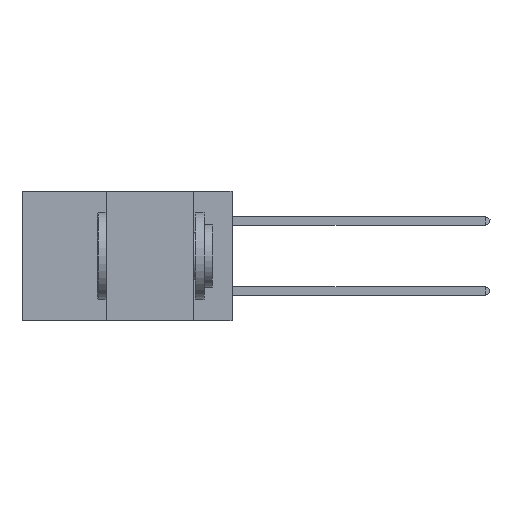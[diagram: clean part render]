
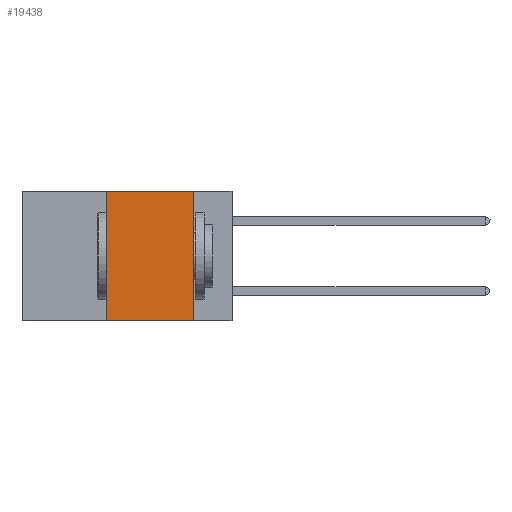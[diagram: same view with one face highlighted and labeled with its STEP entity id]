
A CAD part, left-side view. The second image highlights one B-rep face of the part: STEP entity #19438.
In plain terms, the highlighted planar face has unit normal (-1, 0, 0).
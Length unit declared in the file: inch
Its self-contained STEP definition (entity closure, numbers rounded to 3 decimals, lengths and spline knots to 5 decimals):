
#552 = CARTESIAN_POINT ( 'NONE',  ( 0., 0.11, 0. ) ) ;
#2005 = VERTEX_POINT ( 'NONE', #35096 ) ;
#2149 = VECTOR ( 'NONE', #7782, 39.37008 ) ;
#2191 = EDGE_CURVE ( 'NONE', #21267, #2005, #26869, .T. ) ;
#2265 = DIRECTION ( 'NONE',  ( 0., -1., 0. ) ) ;
#4194 = VECTOR ( 'NONE', #19752, 39.37008 ) ;
#6400 = LINE ( 'NONE', #44155, #4194 ) ;
#6740 = ORIENTED_EDGE ( 'NONE', *, *, #28919, .F. ) ;
#7676 = ORIENTED_EDGE ( 'NONE', *, *, #35363, .F. ) ;
#7782 = DIRECTION ( 'NONE',  ( 0., 0., -1. ) ) ;
#9623 = VECTOR ( 'NONE', #2265, 39.37008 ) ;
#10686 = LINE ( 'NONE', #26790, #9623 ) ;
#11464 = LINE ( 'NONE', #552, #2149 ) ;
#15037 = CARTESIAN_POINT ( 'NONE',  ( 0., 0.36, 0. ) ) ;
#16605 = AXIS2_PLACEMENT_3D ( 'NONE', #36214, #18784, #43182 ) ;
#17268 = VERTEX_POINT ( 'NONE', #19667 ) ;
#18784 = DIRECTION ( 'NONE',  ( 1., 0., 0. ) ) ;
#18826 = CARTESIAN_POINT ( 'NONE',  ( 0., 0.36, -0.37 ) ) ;
#19438 = ADVANCED_FACE ( 'NONE', ( #27217 ), #29230, .F. ) ;
#19667 = CARTESIAN_POINT ( 'NONE',  ( 0., 0.11, 0. ) ) ;
#19752 = DIRECTION ( 'NONE',  ( 0., -1., 0. ) ) ;
#20970 = EDGE_CURVE ( 'NONE', #21267, #39598, #10686, .T. ) ;
#21267 = VERTEX_POINT ( 'NONE', #18826 ) ;
#21929 = DIRECTION ( 'NONE',  ( 0., 0., 1. ) ) ;
#24660 = CARTESIAN_POINT ( 'NONE',  ( 0., 0.11, -0.37 ) ) ;
#25008 = ORIENTED_EDGE ( 'NONE', *, *, #20970, .T. ) ;
#25432 = ORIENTED_EDGE ( 'NONE', *, *, #2191, .F. ) ;
#26790 = CARTESIAN_POINT ( 'NONE',  ( 0., 0.6, -0.37 ) ) ;
#26869 = LINE ( 'NONE', #15037, #35036 ) ;
#27217 = FACE_OUTER_BOUND ( 'NONE', #45080, .T. ) ;
#28919 = EDGE_CURVE ( 'NONE', #17268, #39598, #11464, .T. ) ;
#29230 = PLANE ( 'NONE',  #16605 ) ;
#35036 = VECTOR ( 'NONE', #21929, 39.37008 ) ;
#35096 = CARTESIAN_POINT ( 'NONE',  ( 0., 0.36, 0. ) ) ;
#35363 = EDGE_CURVE ( 'NONE', #2005, #17268, #6400, .T. ) ;
#36214 = CARTESIAN_POINT ( 'NONE',  ( 0., 0.6, 0. ) ) ;
#39598 = VERTEX_POINT ( 'NONE', #24660 ) ;
#43182 = DIRECTION ( 'NONE',  ( 0., 0., -1. ) ) ;
#44155 = CARTESIAN_POINT ( 'NONE',  ( 0., 0.6, 0. ) ) ;
#45080 = EDGE_LOOP ( 'NONE', ( #6740, #7676, #25432, #25008 ) ) ;
